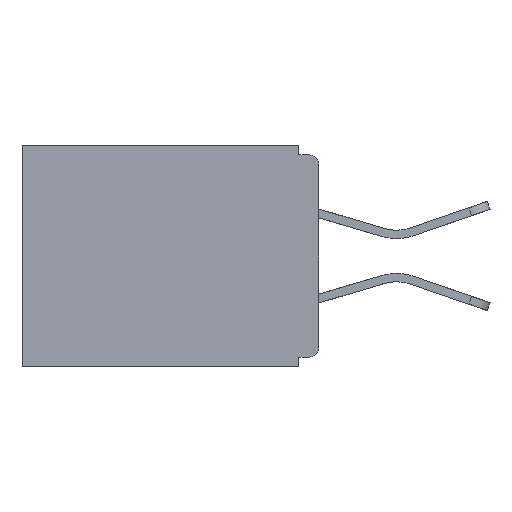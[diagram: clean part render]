
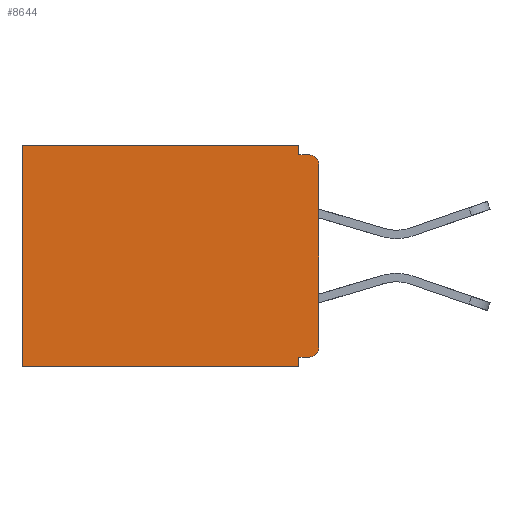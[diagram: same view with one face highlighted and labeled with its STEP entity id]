
A CAD part, left-side view. The second image highlights one B-rep face of the part: STEP entity #8644.
In plain terms, the highlighted planar face has unit normal (-1, 0, 0).
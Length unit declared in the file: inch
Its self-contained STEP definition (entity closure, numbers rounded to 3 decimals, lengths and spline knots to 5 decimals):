
#920 = DIRECTION ( 'NONE',  ( -1., 0., 0. ) ) ;
#970 = VECTOR ( 'NONE', #14046, 39.37008 ) ;
#1956 = VERTEX_POINT ( 'NONE', #4798 ) ;
#2322 = LINE ( 'NONE', #6399, #970 ) ;
#2387 = VECTOR ( 'NONE', #9430, 39.37008 ) ;
#2391 = EDGE_CURVE ( 'NONE', #11975, #13418, #10795, .T. ) ;
#2521 = DIRECTION ( 'NONE',  ( -1., 0., 0. ) ) ;
#2781 = CARTESIAN_POINT ( 'NONE',  ( 0.298, 0.031, -0.343 ) ) ;
#2937 = AXIS2_PLACEMENT_3D ( 'NONE', #13576, #6968, #10262 ) ;
#3163 = EDGE_CURVE ( 'NONE', #3368, #1956, #13349, .T. ) ;
#3368 = VERTEX_POINT ( 'NONE', #7700 ) ;
#3590 = ORIENTED_EDGE ( 'NONE', *, *, #2391, .F. ) ;
#3828 = DIRECTION ( 'NONE',  ( 0., 0., -1. ) ) ;
#3921 = EDGE_CURVE ( 'NONE', #8404, #9982, #10915, .T. ) ;
#3933 = ORIENTED_EDGE ( 'NONE', *, *, #11556, .F. ) ;
#4454 = CARTESIAN_POINT ( 'NONE',  ( 0.298, 0., 0. ) ) ;
#4514 = EDGE_CURVE ( 'NONE', #13502, #8404, #13135, .T. ) ;
#4798 = CARTESIAN_POINT ( 'NONE',  ( 0.298, 0.031, -0.343 ) ) ;
#4860 = VERTEX_POINT ( 'NONE', #11681 ) ;
#4974 = VERTEX_POINT ( 'NONE', #10855 ) ;
#5046 = EDGE_CURVE ( 'NONE', #4974, #3368, #9179, .T. ) ;
#5418 = CARTESIAN_POINT ( 'NONE',  ( 0.298, 0.031, 0. ) ) ;
#5782 = DIRECTION ( 'NONE',  ( 0., 0., -1. ) ) ;
#5873 = CARTESIAN_POINT ( 'NONE',  ( 0.298, 0.46, 0. ) ) ;
#5903 = CIRCLE ( 'NONE', #8532, 0.015 ) ;
#5926 = EDGE_CURVE ( 'NONE', #1956, #9982, #6062, .T. ) ;
#6062 = LINE ( 'NONE', #10239, #10324 ) ;
#6080 = DIRECTION ( 'NONE',  ( 0., 0., -1. ) ) ;
#6104 = PLANE ( 'NONE',  #2937 ) ;
#6242 = CARTESIAN_POINT ( 'NONE',  ( 0.298, 0.46, -0.343 ) ) ;
#6326 = EDGE_CURVE ( 'NONE', #13502, #4860, #2322, .T. ) ;
#6399 = CARTESIAN_POINT ( 'NONE',  ( 0.298, 0.031, -0.343 ) ) ;
#6480 = ORIENTED_EDGE ( 'NONE', *, *, #3163, .F. ) ;
#6499 = VECTOR ( 'NONE', #3828, 39.37008 ) ;
#6622 = LINE ( 'NONE', #7331, #2387 ) ;
#6799 = CARTESIAN_POINT ( 'NONE',  ( 0.298, 0., -0.03 ) ) ;
#6968 = DIRECTION ( 'NONE',  ( 1., 0., 0. ) ) ;
#7134 = DIRECTION ( 'NONE',  ( 0., 1., 0. ) ) ;
#7331 = CARTESIAN_POINT ( 'NONE',  ( 0.298, 0., -0.015 ) ) ;
#7417 = CARTESIAN_POINT ( 'NONE',  ( 0.298, 0.015, -0.03 ) ) ;
#7557 = CARTESIAN_POINT ( 'NONE',  ( 0.298, 0., -0.328 ) ) ;
#7700 = CARTESIAN_POINT ( 'NONE',  ( 0.298, 0.031, -0.328 ) ) ;
#7982 = VERTEX_POINT ( 'NONE', #13027 ) ;
#8204 = EDGE_CURVE ( 'NONE', #11975, #7982, #9077, .T. ) ;
#8404 = VERTEX_POINT ( 'NONE', #13727 ) ;
#8469 = VECTOR ( 'NONE', #9037, 39.37008 ) ;
#8532 = AXIS2_PLACEMENT_3D ( 'NONE', #13352, #2521, #8958 ) ;
#8644 = ADVANCED_FACE ( 'NONE', ( #10248 ), #6104, .F. ) ;
#8868 = VECTOR ( 'NONE', #5782, 39.37008 ) ;
#8958 = DIRECTION ( 'NONE',  ( 0., 0., -1. ) ) ;
#8986 = ORIENTED_EDGE ( 'NONE', *, *, #13093, .T. ) ;
#9037 = DIRECTION ( 'NONE',  ( 0., 1., 0. ) ) ;
#9077 = CIRCLE ( 'NONE', #11340, 0.015 ) ;
#9179 = LINE ( 'NONE', #7557, #8469 ) ;
#9430 = DIRECTION ( 'NONE',  ( 0., -1., 0. ) ) ;
#9982 = VERTEX_POINT ( 'NONE', #6242 ) ;
#9999 = EDGE_LOOP ( 'NONE', ( #13209, #3933, #11525, #13892, #10340, #11510, #6480, #12949, #8986, #3590 ) ) ;
#10212 = VECTOR ( 'NONE', #10941, 39.37008 ) ;
#10239 = CARTESIAN_POINT ( 'NONE',  ( 0.298, 0., -0.343 ) ) ;
#10248 = FACE_OUTER_BOUND ( 'NONE', #9999, .T. ) ;
#10257 = DIRECTION ( 'NONE',  ( 0., 0., -1. ) ) ;
#10262 = DIRECTION ( 'NONE',  ( 0., 0., -1. ) ) ;
#10324 = VECTOR ( 'NONE', #7134, 39.37008 ) ;
#10340 = ORIENTED_EDGE ( 'NONE', *, *, #3921, .T. ) ;
#10608 = CARTESIAN_POINT ( 'NONE',  ( 0.298, 0., -0.313 ) ) ;
#10795 = LINE ( 'NONE', #11278, #11828 ) ;
#10855 = CARTESIAN_POINT ( 'NONE',  ( 0.298, 0.015, -0.328 ) ) ;
#10915 = LINE ( 'NONE', #5873, #8868 ) ;
#10941 = DIRECTION ( 'NONE',  ( 0., 1., 0. ) ) ;
#11278 = CARTESIAN_POINT ( 'NONE',  ( 0.298, 0., 0. ) ) ;
#11340 = AXIS2_PLACEMENT_3D ( 'NONE', #7417, #920, #6080 ) ;
#11510 = ORIENTED_EDGE ( 'NONE', *, *, #5926, .F. ) ;
#11525 = ORIENTED_EDGE ( 'NONE', *, *, #6326, .F. ) ;
#11556 = EDGE_CURVE ( 'NONE', #4860, #7982, #6622, .T. ) ;
#11681 = CARTESIAN_POINT ( 'NONE',  ( 0.298, 0.031, -0.015 ) ) ;
#11828 = VECTOR ( 'NONE', #10257, 39.37008 ) ;
#11975 = VERTEX_POINT ( 'NONE', #6799 ) ;
#12949 = ORIENTED_EDGE ( 'NONE', *, *, #5046, .F. ) ;
#13027 = CARTESIAN_POINT ( 'NONE',  ( 0.298, 0.015, -0.015 ) ) ;
#13093 = EDGE_CURVE ( 'NONE', #4974, #13418, #5903, .T. ) ;
#13135 = LINE ( 'NONE', #4454, #10212 ) ;
#13209 = ORIENTED_EDGE ( 'NONE', *, *, #8204, .T. ) ;
#13349 = LINE ( 'NONE', #2781, #6499 ) ;
#13352 = CARTESIAN_POINT ( 'NONE',  ( 0.298, 0.015, -0.313 ) ) ;
#13418 = VERTEX_POINT ( 'NONE', #10608 ) ;
#13502 = VERTEX_POINT ( 'NONE', #5418 ) ;
#13576 = CARTESIAN_POINT ( 'NONE',  ( 0.298, 0., 0. ) ) ;
#13727 = CARTESIAN_POINT ( 'NONE',  ( 0.298, 0.46, 0. ) ) ;
#13892 = ORIENTED_EDGE ( 'NONE', *, *, #4514, .T. ) ;
#14046 = DIRECTION ( 'NONE',  ( 0., 0., -1. ) ) ;
